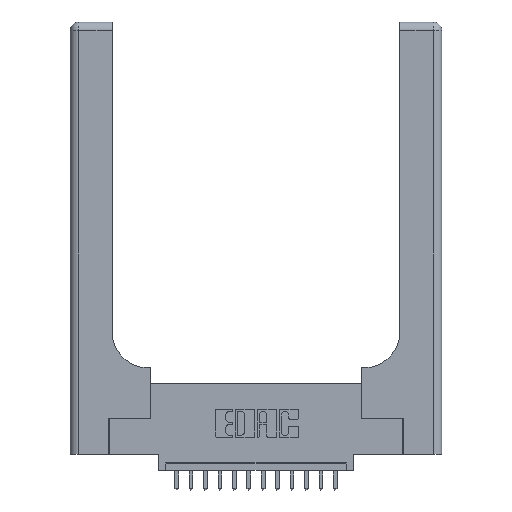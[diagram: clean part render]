
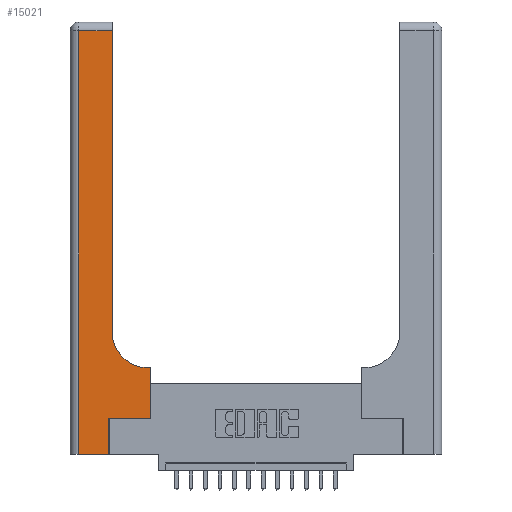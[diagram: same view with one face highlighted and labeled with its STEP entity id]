
A CAD part, top view. The second image highlights one B-rep face of the part: STEP entity #15021.
In plain terms, the highlighted planar face has unit normal (0, 0, 1).
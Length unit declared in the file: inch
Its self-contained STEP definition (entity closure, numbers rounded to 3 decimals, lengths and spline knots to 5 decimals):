
#241 = CARTESIAN_POINT ( 'NONE',  ( 0.5415, 0.85, 0.37 ) ) ;
#430 = ORIENTED_EDGE ( 'NONE', *, *, #15331, .T. ) ;
#624 = EDGE_CURVE ( 'NONE', #3422, #1430, #17321, .T. ) ;
#631 = DIRECTION ( 'NONE',  ( -1., 0., 0. ) ) ;
#769 = ORIENTED_EDGE ( 'NONE', *, *, #3098, .T. ) ;
#921 = VERTEX_POINT ( 'NONE', #1110 ) ;
#1110 = CARTESIAN_POINT ( 'NONE',  ( 0.06, 2.94, 0.37 ) ) ;
#1430 = VERTEX_POINT ( 'NONE', #13429 ) ;
#2737 = LINE ( 'NONE', #10116, #6313 ) ;
#2765 = VECTOR ( 'NONE', #631, 39.37008 ) ;
#2902 = EDGE_CURVE ( 'NONE', #6879, #3422, #3211, .T. ) ;
#3098 = EDGE_CURVE ( 'NONE', #8236, #10852, #6122, .T. ) ;
#3211 = LINE ( 'NONE', #5184, #14554 ) ;
#3422 = VERTEX_POINT ( 'NONE', #10131 ) ;
#4009 = CARTESIAN_POINT ( 'NONE',  ( 0., 3., 0.37 ) ) ;
#4018 = VECTOR ( 'NONE', #14112, 39.37008 ) ;
#4209 = EDGE_CURVE ( 'NONE', #6717, #8236, #8945, .T. ) ;
#4385 = LINE ( 'NONE', #10360, #12802 ) ;
#4821 = ORIENTED_EDGE ( 'NONE', *, *, #2902, .T. ) ;
#5160 = ORIENTED_EDGE ( 'NONE', *, *, #4209, .T. ) ;
#5184 = CARTESIAN_POINT ( 'NONE',  ( 0., 0., 0.37 ) ) ;
#5217 = VERTEX_POINT ( 'NONE', #17109 ) ;
#6069 = DIRECTION ( 'NONE',  ( 0., 0., -1. ) ) ;
#6122 = CIRCLE ( 'NONE', #8971, 0.25 ) ;
#6138 = DIRECTION ( 'NONE',  ( 1., 0., 0. ) ) ;
#6313 = VECTOR ( 'NONE', #8644, 39.37008 ) ;
#6662 = ORIENTED_EDGE ( 'NONE', *, *, #624, .T. ) ;
#6717 = VERTEX_POINT ( 'NONE', #17277 ) ;
#6831 = CARTESIAN_POINT ( 'NONE',  ( 0.5415, 0.6, 0.37 ) ) ;
#6879 = VERTEX_POINT ( 'NONE', #7396 ) ;
#7044 = DIRECTION ( 'NONE',  ( 0., 0., -1. ) ) ;
#7396 = CARTESIAN_POINT ( 'NONE',  ( 0.06, 0., 0.37 ) ) ;
#7414 = DIRECTION ( 'NONE',  ( 0., 1., 0. ) ) ;
#7908 = CARTESIAN_POINT ( 'NONE',  ( 0.269, 0.25, 0.37 ) ) ;
#7939 = FACE_OUTER_BOUND ( 'NONE', #8436, .T. ) ;
#8236 = VERTEX_POINT ( 'NONE', #6831 ) ;
#8436 = EDGE_LOOP ( 'NONE', ( #10703, #12418, #13344, #4821, #6662, #12706, #430, #5160, #769 ) ) ;
#8644 = DIRECTION ( 'NONE',  ( 0., 1., 0. ) ) ;
#8945 = LINE ( 'NONE', #9517, #15635 ) ;
#8971 = AXIS2_PLACEMENT_3D ( 'NONE', #241, #6069, #6138 ) ;
#9103 = LINE ( 'NONE', #16936, #4018 ) ;
#9517 = CARTESIAN_POINT ( 'NONE',  ( 0.2915, 0.6, 0.37 ) ) ;
#9884 = CARTESIAN_POINT ( 'NONE',  ( 0.269, 0., 0.37 ) ) ;
#10116 = CARTESIAN_POINT ( 'NONE',  ( 0.2915, 3., 0.37 ) ) ;
#10131 = CARTESIAN_POINT ( 'NONE',  ( 0.269, 0., 0.37 ) ) ;
#10337 = DIRECTION ( 'NONE',  ( -1., 0., 0. ) ) ;
#10360 = CARTESIAN_POINT ( 'NONE',  ( 0.5585, 0.25, 0.37 ) ) ;
#10703 = ORIENTED_EDGE ( 'NONE', *, *, #18153, .T. ) ;
#10852 = VERTEX_POINT ( 'NONE', #10897 ) ;
#10863 = VECTOR ( 'NONE', #7414, 39.37008 ) ;
#10897 = CARTESIAN_POINT ( 'NONE',  ( 0.2915, 0.85, 0.37 ) ) ;
#11663 = VERTEX_POINT ( 'NONE', #15840 ) ;
#12418 = ORIENTED_EDGE ( 'NONE', *, *, #17209, .T. ) ;
#12706 = ORIENTED_EDGE ( 'NONE', *, *, #13211, .T. ) ;
#12802 = VECTOR ( 'NONE', #13345, 39.37008 ) ;
#12994 = AXIS2_PLACEMENT_3D ( 'NONE', #4009, #7044, #16864 ) ;
#13095 = VECTOR ( 'NONE', #17862, 39.37008 ) ;
#13189 = LINE ( 'NONE', #17584, #2765 ) ;
#13211 = EDGE_CURVE ( 'NONE', #1430, #5217, #15994, .T. ) ;
#13344 = ORIENTED_EDGE ( 'NONE', *, *, #13453, .T. ) ;
#13345 = DIRECTION ( 'NONE',  ( 0., 1., 0. ) ) ;
#13429 = CARTESIAN_POINT ( 'NONE',  ( 0.269, 0.25, 0.37 ) ) ;
#13453 = EDGE_CURVE ( 'NONE', #921, #6879, #9103, .T. ) ;
#13918 = PLANE ( 'NONE',  #12994 ) ;
#14112 = DIRECTION ( 'NONE',  ( 0., -1., 0. ) ) ;
#14554 = VECTOR ( 'NONE', #17976, 39.37008 ) ;
#15021 = ADVANCED_FACE ( 'NONE', ( #7939 ), #13918, .F. ) ;
#15331 = EDGE_CURVE ( 'NONE', #5217, #6717, #4385, .T. ) ;
#15635 = VECTOR ( 'NONE', #10337, 39.37008 ) ;
#15840 = CARTESIAN_POINT ( 'NONE',  ( 0.2915, 2.94, 0.37 ) ) ;
#15994 = LINE ( 'NONE', #7908, #13095 ) ;
#16864 = DIRECTION ( 'NONE',  ( -1., 0., 0. ) ) ;
#16936 = CARTESIAN_POINT ( 'NONE',  ( 0.06, 3., 0.37 ) ) ;
#17109 = CARTESIAN_POINT ( 'NONE',  ( 0.5585, 0.25, 0.37 ) ) ;
#17209 = EDGE_CURVE ( 'NONE', #11663, #921, #13189, .T. ) ;
#17277 = CARTESIAN_POINT ( 'NONE',  ( 0.5585, 0.6, 0.37 ) ) ;
#17321 = LINE ( 'NONE', #9884, #10863 ) ;
#17584 = CARTESIAN_POINT ( 'NONE',  ( 0., 2.94, 0.37 ) ) ;
#17862 = DIRECTION ( 'NONE',  ( 1., 0., 0. ) ) ;
#17976 = DIRECTION ( 'NONE',  ( 1., 0., 0. ) ) ;
#18153 = EDGE_CURVE ( 'NONE', #10852, #11663, #2737, .T. ) ;
